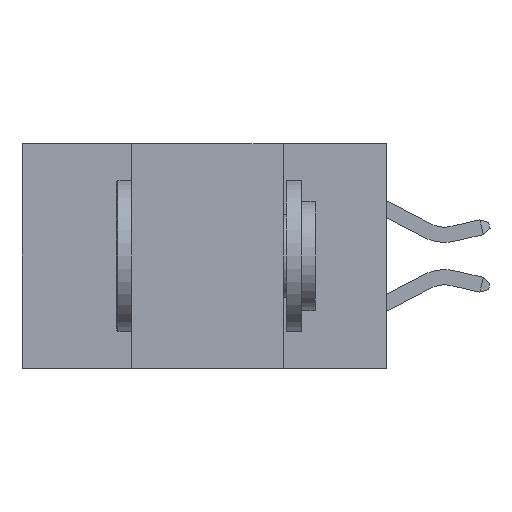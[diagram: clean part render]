
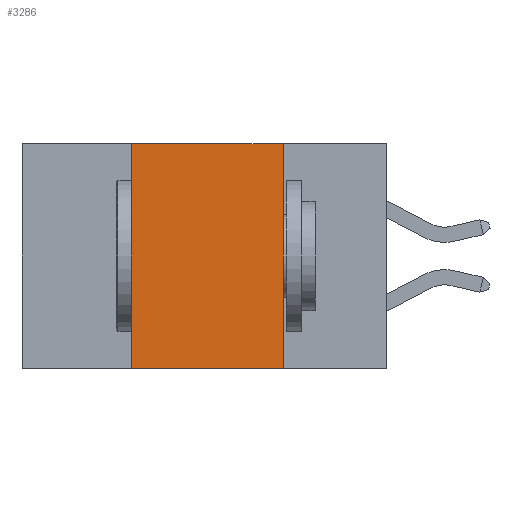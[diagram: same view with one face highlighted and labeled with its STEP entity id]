
A CAD part, left-side view. The second image highlights one B-rep face of the part: STEP entity #3286.
In plain terms, the highlighted planar face has unit normal (-1, 0, 0).
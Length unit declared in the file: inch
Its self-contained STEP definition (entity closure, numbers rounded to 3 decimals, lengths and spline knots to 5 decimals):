
#185 = CARTESIAN_POINT ( 'NONE',  ( 0., 0.6, -0.37 ) ) ;
#237 = ORIENTED_EDGE ( 'NONE', *, *, #7846, .F. ) ;
#613 = ORIENTED_EDGE ( 'NONE', *, *, #13984, .F. ) ;
#2003 = PLANE ( 'NONE',  #15421 ) ;
#2211 = LINE ( 'NONE', #185, #15884 ) ;
#2460 = LINE ( 'NONE', #15882, #2861 ) ;
#2861 = VECTOR ( 'NONE', #11011, 39.37008 ) ;
#3072 = LINE ( 'NONE', #9219, #15955 ) ;
#3286 = ADVANCED_FACE ( 'NONE', ( #4915 ), #2003, .F. ) ;
#3742 = CARTESIAN_POINT ( 'NONE',  ( 0., 0.17, -0.37 ) ) ;
#3951 = ORIENTED_EDGE ( 'NONE', *, *, #7523, .T. ) ;
#4009 = CARTESIAN_POINT ( 'NONE',  ( 0., 0.42, 0. ) ) ;
#4583 = EDGE_CURVE ( 'NONE', #11728, #8676, #3072, .T. ) ;
#4915 = FACE_OUTER_BOUND ( 'NONE', #6980, .T. ) ;
#5219 = VERTEX_POINT ( 'NONE', #3742 ) ;
#6105 = CARTESIAN_POINT ( 'NONE',  ( 0., 0.17, 0. ) ) ;
#6940 = ORIENTED_EDGE ( 'NONE', *, *, #4583, .F. ) ;
#6980 = EDGE_LOOP ( 'NONE', ( #237, #6940, #613, #3951 ) ) ;
#7523 = EDGE_CURVE ( 'NONE', #11691, #5219, #2211, .T. ) ;
#7582 = VECTOR ( 'NONE', #10892, 39.37008 ) ;
#7828 = CARTESIAN_POINT ( 'NONE',  ( 0., 0.42, -0.37 ) ) ;
#7846 = EDGE_CURVE ( 'NONE', #8676, #5219, #10943, .T. ) ;
#8361 = CARTESIAN_POINT ( 'NONE',  ( 0., 0.17, 0. ) ) ;
#8676 = VERTEX_POINT ( 'NONE', #6105 ) ;
#9051 = DIRECTION ( 'NONE',  ( 0., -1., 0. ) ) ;
#9219 = CARTESIAN_POINT ( 'NONE',  ( 0., 0.6, 0. ) ) ;
#10892 = DIRECTION ( 'NONE',  ( 0., 0., -1. ) ) ;
#10943 = LINE ( 'NONE', #8361, #7582 ) ;
#11011 = DIRECTION ( 'NONE',  ( 0., 0., 1. ) ) ;
#11691 = VERTEX_POINT ( 'NONE', #7828 ) ;
#11728 = VERTEX_POINT ( 'NONE', #4009 ) ;
#11872 = DIRECTION ( 'NONE',  ( 0., -1., 0. ) ) ;
#12051 = CARTESIAN_POINT ( 'NONE',  ( 0., 0.6, 0. ) ) ;
#13107 = DIRECTION ( 'NONE',  ( 1., 0., 0. ) ) ;
#13174 = DIRECTION ( 'NONE',  ( 0., 0., -1. ) ) ;
#13984 = EDGE_CURVE ( 'NONE', #11691, #11728, #2460, .T. ) ;
#15421 = AXIS2_PLACEMENT_3D ( 'NONE', #12051, #13107, #13174 ) ;
#15882 = CARTESIAN_POINT ( 'NONE',  ( 0., 0.42, 0. ) ) ;
#15884 = VECTOR ( 'NONE', #9051, 39.37008 ) ;
#15955 = VECTOR ( 'NONE', #11872, 39.37008 ) ;
